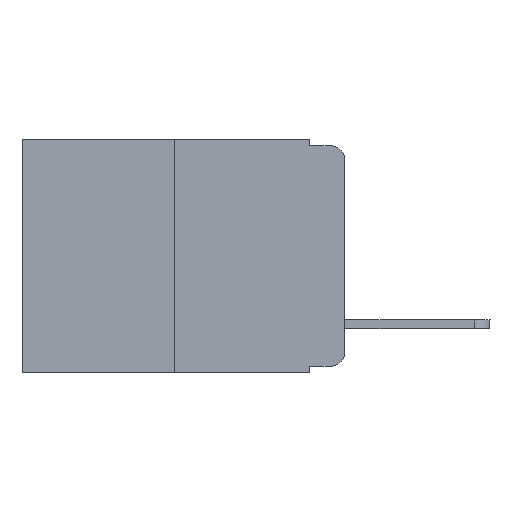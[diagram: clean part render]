
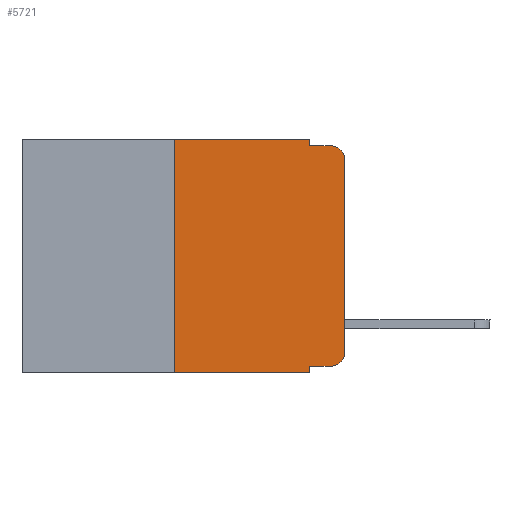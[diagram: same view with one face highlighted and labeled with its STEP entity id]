
A CAD part, left-side view. The second image highlights one B-rep face of the part: STEP entity #5721.
In plain terms, the highlighted planar face has unit normal (-1, 0, 0).
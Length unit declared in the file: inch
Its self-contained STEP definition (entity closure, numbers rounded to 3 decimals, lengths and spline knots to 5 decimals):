
#154 = AXIS2_PLACEMENT_3D ( 'NONE', #4279, #10916, #2443 ) ;
#617 = VERTEX_POINT ( 'NONE', #4067 ) ;
#636 = ORIENTED_EDGE ( 'NONE', *, *, #5229, .F. ) ;
#736 = EDGE_CURVE ( 'NONE', #6299, #6843, #2243, .T. ) ;
#868 = CARTESIAN_POINT ( 'NONE',  ( 0., 0.051, -0.333 ) ) ;
#932 = DIRECTION ( 'NONE',  ( 0., -1., 0. ) ) ;
#965 = CARTESIAN_POINT ( 'NONE',  ( 0., 0.02, -0.333 ) ) ;
#1418 = DIRECTION ( 'NONE',  ( 0., 0., -1. ) ) ;
#1661 = CARTESIAN_POINT ( 'NONE',  ( 0., 0.02, -0.313 ) ) ;
#1709 = EDGE_CURVE ( 'NONE', #6843, #617, #8194, .T. ) ;
#1733 = CARTESIAN_POINT ( 'NONE',  ( 0., 0.25, -0.343 ) ) ;
#1938 = CARTESIAN_POINT ( 'NONE',  ( 0., 0., -0.03 ) ) ;
#1969 = VECTOR ( 'NONE', #3891, 39.37008 ) ;
#2243 = LINE ( 'NONE', #9790, #2971 ) ;
#2246 = VERTEX_POINT ( 'NONE', #10270 ) ;
#2310 = DIRECTION ( 'NONE',  ( 0., 0., 1. ) ) ;
#2400 = CARTESIAN_POINT ( 'NONE',  ( 0., 0.051, -0.01 ) ) ;
#2443 = DIRECTION ( 'NONE',  ( 0., 0., -1. ) ) ;
#2676 = EDGE_CURVE ( 'NONE', #3654, #617, #6091, .T. ) ;
#2858 = EDGE_CURVE ( 'NONE', #10216, #2246, #11741, .T. ) ;
#2945 = VECTOR ( 'NONE', #8627, 39.37008 ) ;
#2970 = CARTESIAN_POINT ( 'NONE',  ( 0., 0.051, -0.01 ) ) ;
#2971 = VECTOR ( 'NONE', #2310, 39.37008 ) ;
#3130 = LINE ( 'NONE', #11890, #10523 ) ;
#3177 = VECTOR ( 'NONE', #7079, 39.37008 ) ;
#3654 = VERTEX_POINT ( 'NONE', #2400 ) ;
#3760 = CARTESIAN_POINT ( 'NONE',  ( 0., 0., -0.313 ) ) ;
#3891 = DIRECTION ( 'NONE',  ( 0., 0., -1. ) ) ;
#4067 = CARTESIAN_POINT ( 'NONE',  ( 0., 0.02, -0.01 ) ) ;
#4156 = LINE ( 'NONE', #9465, #7363 ) ;
#4279 = CARTESIAN_POINT ( 'NONE',  ( 0., 0.473, 0. ) ) ;
#4533 = DIRECTION ( 'NONE',  ( -1., 0., 0. ) ) ;
#4697 = AXIS2_PLACEMENT_3D ( 'NONE', #1661, #11214, #7891 ) ;
#4891 = ORIENTED_EDGE ( 'NONE', *, *, #7760, .F. ) ;
#5120 = VERTEX_POINT ( 'NONE', #965 ) ;
#5223 = CARTESIAN_POINT ( 'NONE',  ( 0., 0.25, 0. ) ) ;
#5229 = EDGE_CURVE ( 'NONE', #10730, #11737, #7466, .T. ) ;
#5424 = ORIENTED_EDGE ( 'NONE', *, *, #2858, .F. ) ;
#5721 = ADVANCED_FACE ( 'NONE', ( #12045 ), #9784, .F. ) ;
#6074 = EDGE_CURVE ( 'NONE', #10216, #5120, #7221, .T. ) ;
#6091 = LINE ( 'NONE', #2970, #3177 ) ;
#6117 = EDGE_CURVE ( 'NONE', #11793, #2246, #3130, .T. ) ;
#6133 = CARTESIAN_POINT ( 'NONE',  ( 0., 0.473, 0. ) ) ;
#6299 = VERTEX_POINT ( 'NONE', #3760 ) ;
#6593 = DIRECTION ( 'NONE',  ( 0., -1., 0. ) ) ;
#6682 = VECTOR ( 'NONE', #11711, 39.37008 ) ;
#6843 = VERTEX_POINT ( 'NONE', #1938 ) ;
#6844 = AXIS2_PLACEMENT_3D ( 'NONE', #11035, #4533, #1418 ) ;
#7079 = DIRECTION ( 'NONE',  ( 0., -1., 0. ) ) ;
#7199 = ORIENTED_EDGE ( 'NONE', *, *, #8413, .T. ) ;
#7221 = LINE ( 'NONE', #868, #13909 ) ;
#7363 = VECTOR ( 'NONE', #13770, 39.37008 ) ;
#7466 = LINE ( 'NONE', #6133, #6682 ) ;
#7760 = EDGE_CURVE ( 'NONE', #11793, #10730, #4156, .T. ) ;
#7891 = DIRECTION ( 'NONE',  ( 0., 0., -1. ) ) ;
#8194 = CIRCLE ( 'NONE', #6844, 0.02 ) ;
#8214 = ORIENTED_EDGE ( 'NONE', *, *, #6074, .T. ) ;
#8413 = EDGE_CURVE ( 'NONE', #5120, #6299, #12800, .T. ) ;
#8627 = DIRECTION ( 'NONE',  ( 0., 0., -1. ) ) ;
#9143 = ORIENTED_EDGE ( 'NONE', *, *, #736, .T. ) ;
#9327 = LINE ( 'NONE', #9462, #1969 ) ;
#9462 = CARTESIAN_POINT ( 'NONE',  ( 0., 0.051, 0. ) ) ;
#9465 = CARTESIAN_POINT ( 'NONE',  ( 0., 0.25, 0. ) ) ;
#9494 = ORIENTED_EDGE ( 'NONE', *, *, #11430, .F. ) ;
#9784 = PLANE ( 'NONE',  #154 ) ;
#9790 = CARTESIAN_POINT ( 'NONE',  ( 0., 0., 0. ) ) ;
#10213 = CARTESIAN_POINT ( 'NONE',  ( 0., 0.051, 0. ) ) ;
#10216 = VERTEX_POINT ( 'NONE', #13382 ) ;
#10270 = CARTESIAN_POINT ( 'NONE',  ( 0., 0.051, -0.343 ) ) ;
#10523 = VECTOR ( 'NONE', #6593, 39.37008 ) ;
#10730 = VERTEX_POINT ( 'NONE', #5223 ) ;
#10916 = DIRECTION ( 'NONE',  ( 1., 0., 0. ) ) ;
#11035 = CARTESIAN_POINT ( 'NONE',  ( 0., 0.02, -0.03 ) ) ;
#11214 = DIRECTION ( 'NONE',  ( -1., 0., 0. ) ) ;
#11362 = ORIENTED_EDGE ( 'NONE', *, *, #6117, .T. ) ;
#11430 = EDGE_CURVE ( 'NONE', #11737, #3654, #9327, .T. ) ;
#11711 = DIRECTION ( 'NONE',  ( 0., -1., 0. ) ) ;
#11737 = VERTEX_POINT ( 'NONE', #10213 ) ;
#11741 = LINE ( 'NONE', #13849, #2945 ) ;
#11793 = VERTEX_POINT ( 'NONE', #1733 ) ;
#11890 = CARTESIAN_POINT ( 'NONE',  ( 0., 0.473, -0.343 ) ) ;
#12045 = FACE_OUTER_BOUND ( 'NONE', #12096, .T. ) ;
#12096 = EDGE_LOOP ( 'NONE', ( #9143, #12693, #12478, #9494, #636, #4891, #11362, #5424, #8214, #7199 ) ) ;
#12478 = ORIENTED_EDGE ( 'NONE', *, *, #2676, .F. ) ;
#12693 = ORIENTED_EDGE ( 'NONE', *, *, #1709, .T. ) ;
#12800 = CIRCLE ( 'NONE', #4697, 0.02 ) ;
#13382 = CARTESIAN_POINT ( 'NONE',  ( 0., 0.051, -0.333 ) ) ;
#13770 = DIRECTION ( 'NONE',  ( 0., 0., 1. ) ) ;
#13849 = CARTESIAN_POINT ( 'NONE',  ( 0., 0.051, 0. ) ) ;
#13909 = VECTOR ( 'NONE', #932, 39.37008 ) ;
